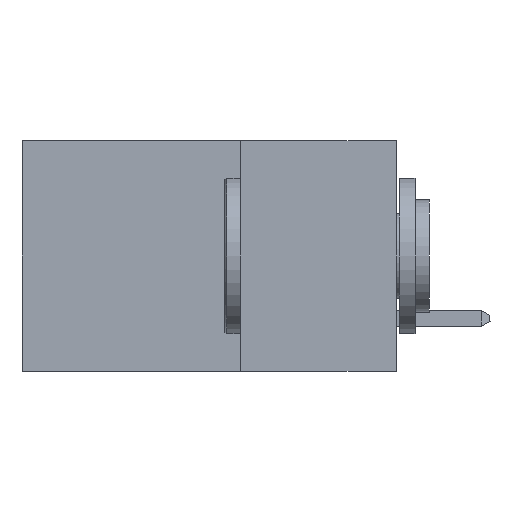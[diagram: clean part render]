
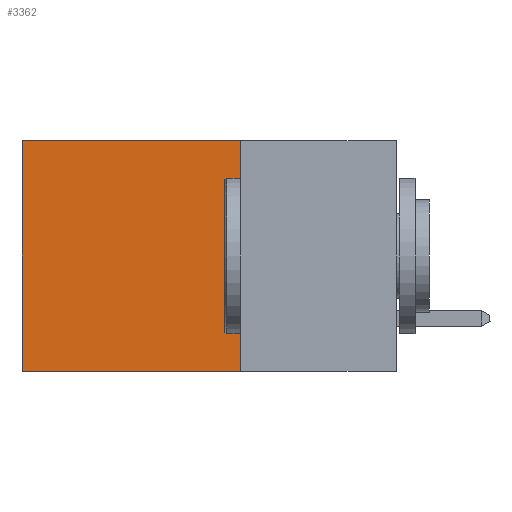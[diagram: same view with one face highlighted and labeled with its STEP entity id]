
A CAD part, left-side view. The second image highlights one B-rep face of the part: STEP entity #3362.
In plain terms, the highlighted planar face has unit normal (-1, 0, 0).
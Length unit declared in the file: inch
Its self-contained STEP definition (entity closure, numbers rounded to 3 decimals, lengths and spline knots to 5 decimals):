
#1007 = CARTESIAN_POINT ( 'NONE',  ( 0.298, 0.6, 0. ) ) ;
#1181 = DIRECTION ( 'NONE',  ( 0., 0., -1. ) ) ;
#1246 = DIRECTION ( 'NONE',  ( 1., 0., 0. ) ) ;
#1589 = EDGE_CURVE ( 'NONE', #15051, #3634, #18324, .T. ) ;
#1805 = VECTOR ( 'NONE', #19335, 39.37008 ) ;
#2574 = VERTEX_POINT ( 'NONE', #1007 ) ;
#2590 = CARTESIAN_POINT ( 'NONE',  ( 0.298, 0.25, 0. ) ) ;
#2626 = CARTESIAN_POINT ( 'NONE',  ( 0.298, 0.25, 0. ) ) ;
#3035 = EDGE_CURVE ( 'NONE', #2574, #3634, #18499, .T. ) ;
#3274 = CARTESIAN_POINT ( 'NONE',  ( 0.298, 0.25, 0. ) ) ;
#3346 = ORIENTED_EDGE ( 'NONE', *, *, #5265, .F. ) ;
#3362 = ADVANCED_FACE ( 'NONE', ( #6330 ), #19070, .F. ) ;
#3634 = VERTEX_POINT ( 'NONE', #17270 ) ;
#4039 = DIRECTION ( 'NONE',  ( 0., 1., 0. ) ) ;
#5265 = EDGE_CURVE ( 'NONE', #17586, #15051, #18869, .T. ) ;
#5448 = VECTOR ( 'NONE', #6018, 39.37008 ) ;
#6018 = DIRECTION ( 'NONE',  ( 0., 1., 0. ) ) ;
#6330 = FACE_OUTER_BOUND ( 'NONE', #15875, .T. ) ;
#6622 = EDGE_CURVE ( 'NONE', #17586, #2574, #9770, .T. ) ;
#8001 = VECTOR ( 'NONE', #14974, 39.37008 ) ;
#8818 = VECTOR ( 'NONE', #4039, 39.37008 ) ;
#9770 = LINE ( 'NONE', #2590, #8818 ) ;
#11292 = CARTESIAN_POINT ( 'NONE',  ( 0.298, 0.6, 0. ) ) ;
#14348 = ORIENTED_EDGE ( 'NONE', *, *, #6622, .T. ) ;
#14974 = DIRECTION ( 'NONE',  ( 0., 0., -1. ) ) ;
#15051 = VERTEX_POINT ( 'NONE', #15090 ) ;
#15074 = CARTESIAN_POINT ( 'NONE',  ( 0.298, 0.25, -0.37 ) ) ;
#15090 = CARTESIAN_POINT ( 'NONE',  ( 0.298, 0.25, -0.37 ) ) ;
#15875 = EDGE_LOOP ( 'NONE', ( #15895, #17563, #3346, #14348 ) ) ;
#15895 = ORIENTED_EDGE ( 'NONE', *, *, #3035, .T. ) ;
#16119 = CARTESIAN_POINT ( 'NONE',  ( 0.298, 0.25, 0. ) ) ;
#17270 = CARTESIAN_POINT ( 'NONE',  ( 0.298, 0.6, -0.37 ) ) ;
#17563 = ORIENTED_EDGE ( 'NONE', *, *, #1589, .F. ) ;
#17586 = VERTEX_POINT ( 'NONE', #3274 ) ;
#18324 = LINE ( 'NONE', #15074, #5448 ) ;
#18499 = LINE ( 'NONE', #11292, #8001 ) ;
#18869 = LINE ( 'NONE', #16119, #1805 ) ;
#19070 = PLANE ( 'NONE',  #19400 ) ;
#19335 = DIRECTION ( 'NONE',  ( 0., 0., -1. ) ) ;
#19400 = AXIS2_PLACEMENT_3D ( 'NONE', #2626, #1246, #1181 ) ;
